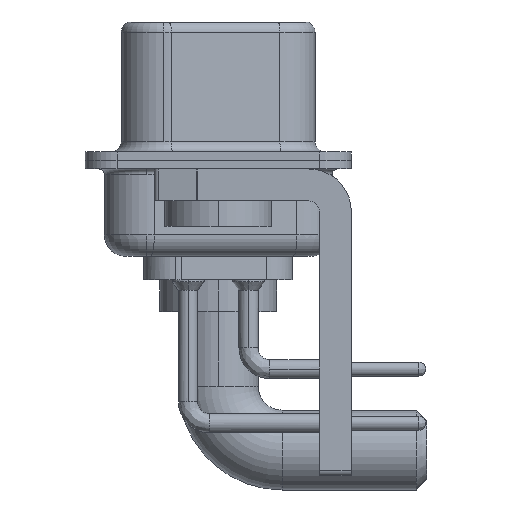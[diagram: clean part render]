
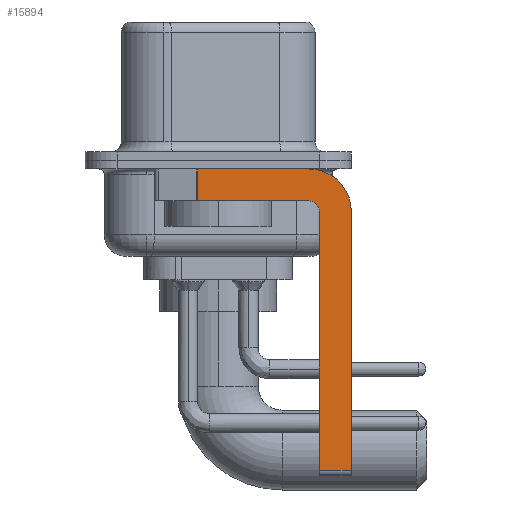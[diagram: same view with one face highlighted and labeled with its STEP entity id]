
A CAD part, left-side view. The second image highlights one B-rep face of the part: STEP entity #15894.
In plain terms, the highlighted planar face has unit normal (-1, 0, 0).
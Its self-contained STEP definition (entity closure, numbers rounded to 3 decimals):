
#106 = ORIENTED_EDGE ( 'NONE', *, *, #12822, .F. ) ;
#1160 = ORIENTED_EDGE ( 'NONE', *, *, #17742, .T. ) ;
#1937 = CARTESIAN_POINT ( 'NONE',  ( -2.9, -4.25, -14.55 ) ) ;
#2468 = VECTOR ( 'NONE', #10219, 1000. ) ;
#2583 = ORIENTED_EDGE ( 'NONE', *, *, #11483, .F. ) ;
#3040 = EDGE_CURVE ( 'NONE', #13359, #24754, #17176, .T. ) ;
#3460 = DIRECTION ( 'NONE',  ( 0., -1., 0. ) ) ;
#3708 = DIRECTION ( 'NONE',  ( 0., 0., 1. ) ) ;
#3843 = DIRECTION ( 'NONE',  ( 0., 0., -1. ) ) ;
#3868 = DIRECTION ( 'NONE',  ( 1., 0., 0. ) ) ;
#3973 = DIRECTION ( 'NONE',  ( -1., 0., 0. ) ) ;
#5087 = CARTESIAN_POINT ( 'NONE',  ( -2.9, -4.25, -2.4 ) ) ;
#5359 = DIRECTION ( 'NONE',  ( 1., 0., 0. ) ) ;
#5526 = ORIENTED_EDGE ( 'NONE', *, *, #3040, .F. ) ;
#5637 = LINE ( 'NONE', #6158, #15110 ) ;
#5878 = CARTESIAN_POINT ( 'NONE',  ( -2.9, 0.978, -1.9 ) ) ;
#5905 = CARTESIAN_POINT ( 'NONE',  ( -2.9, -4.25, -2.4 ) ) ;
#6158 = CARTESIAN_POINT ( 'NONE',  ( -2.9, 3., -0.4 ) ) ;
#6272 = EDGE_CURVE ( 'NONE', #24754, #26449, #13408, .T. ) ;
#6919 = LINE ( 'NONE', #10974, #9427 ) ;
#7082 = EDGE_CURVE ( 'NONE', #18602, #14772, #12143, .T. ) ;
#8034 = LINE ( 'NONE', #5878, #17849 ) ;
#9427 = VECTOR ( 'NONE', #17334, 1000. ) ;
#9582 = VERTEX_POINT ( 'NONE', #25114 ) ;
#9694 = PLANE ( 'NONE',  #22845 ) ;
#9896 = AXIS2_PLACEMENT_3D ( 'NONE', #5087, #5359, #13625 ) ;
#10001 = VERTEX_POINT ( 'NONE', #12483 ) ;
#10219 = DIRECTION ( 'NONE',  ( 0., -1., 0. ) ) ;
#10852 = ORIENTED_EDGE ( 'NONE', *, *, #25193, .F. ) ;
#10974 = CARTESIAN_POINT ( 'NONE',  ( -2.9, -4.75, -14.8 ) ) ;
#11235 = CARTESIAN_POINT ( 'NONE',  ( -2.9, -4.75, -14.55 ) ) ;
#11483 = EDGE_CURVE ( 'NONE', #9582, #18011, #13368, .T. ) ;
#11583 = CARTESIAN_POINT ( 'NONE',  ( -2.9, -6.25, -2.4 ) ) ;
#12109 = CARTESIAN_POINT ( 'NONE',  ( -2.9, -6.25, -14.55 ) ) ;
#12126 = VECTOR ( 'NONE', #19983, 1000. ) ;
#12131 = ORIENTED_EDGE ( 'NONE', *, *, #16449, .F. ) ;
#12143 = LINE ( 'NONE', #1937, #2468 ) ;
#12483 = CARTESIAN_POINT ( 'NONE',  ( -2.9, 0.978, -0.4 ) ) ;
#12486 = VECTOR ( 'NONE', #23314, 1000. ) ;
#12822 = EDGE_CURVE ( 'NONE', #18011, #14772, #24201, .T. ) ;
#13359 = VERTEX_POINT ( 'NONE', #22002 ) ;
#13368 = CIRCLE ( 'NONE', #9896, 2. ) ;
#13408 = LINE ( 'NONE', #21151, #12486 ) ;
#13625 = DIRECTION ( 'NONE',  ( 0., 0., -1. ) ) ;
#14772 = VERTEX_POINT ( 'NONE', #12109 ) ;
#15110 = VECTOR ( 'NONE', #3460, 1000. ) ;
#15894 = ADVANCED_FACE ( 'NONE', ( #16827 ), #9694, .F. ) ;
#16449 = EDGE_CURVE ( 'NONE', #18602, #13359, #6919, .T. ) ;
#16827 = FACE_OUTER_BOUND ( 'NONE', #17278, .T. ) ;
#16945 = ORIENTED_EDGE ( 'NONE', *, *, #6272, .F. ) ;
#17176 = CIRCLE ( 'NONE', #20215, 0.5 ) ;
#17278 = EDGE_LOOP ( 'NONE', ( #10852, #1160, #16945, #5526, #12131, #19804, #106, #2583 ) ) ;
#17334 = DIRECTION ( 'NONE',  ( 0., 0., 1. ) ) ;
#17691 = CARTESIAN_POINT ( 'NONE',  ( -2.9, -6.25, -2.4 ) ) ;
#17742 = EDGE_CURVE ( 'NONE', #10001, #26449, #8034, .T. ) ;
#17849 = VECTOR ( 'NONE', #3843, 1000. ) ;
#18011 = VERTEX_POINT ( 'NONE', #11583 ) ;
#18602 = VERTEX_POINT ( 'NONE', #11235 ) ;
#19804 = ORIENTED_EDGE ( 'NONE', *, *, #7082, .T. ) ;
#19983 = DIRECTION ( 'NONE',  ( 0., 0., -1. ) ) ;
#20215 = AXIS2_PLACEMENT_3D ( 'NONE', #22419, #3973, #3708 ) ;
#20769 = DIRECTION ( 'NONE',  ( 0., 0., -1. ) ) ;
#21151 = CARTESIAN_POINT ( 'NONE',  ( -2.9, -4.25, -1.9 ) ) ;
#22002 = CARTESIAN_POINT ( 'NONE',  ( -2.9, -4.75, -2.4 ) ) ;
#22419 = CARTESIAN_POINT ( 'NONE',  ( -2.9, -4.25, -2.4 ) ) ;
#22845 = AXIS2_PLACEMENT_3D ( 'NONE', #5905, #3868, #20769 ) ;
#23314 = DIRECTION ( 'NONE',  ( 0., 1., 0. ) ) ;
#23932 = CARTESIAN_POINT ( 'NONE',  ( -2.9, 0.978, -1.9 ) ) ;
#24201 = LINE ( 'NONE', #17691, #12126 ) ;
#24754 = VERTEX_POINT ( 'NONE', #26661 ) ;
#25114 = CARTESIAN_POINT ( 'NONE',  ( -2.9, -4.25, -0.4 ) ) ;
#25193 = EDGE_CURVE ( 'NONE', #10001, #9582, #5637, .T. ) ;
#26449 = VERTEX_POINT ( 'NONE', #23932 ) ;
#26661 = CARTESIAN_POINT ( 'NONE',  ( -2.9, -4.25, -1.9 ) ) ;
